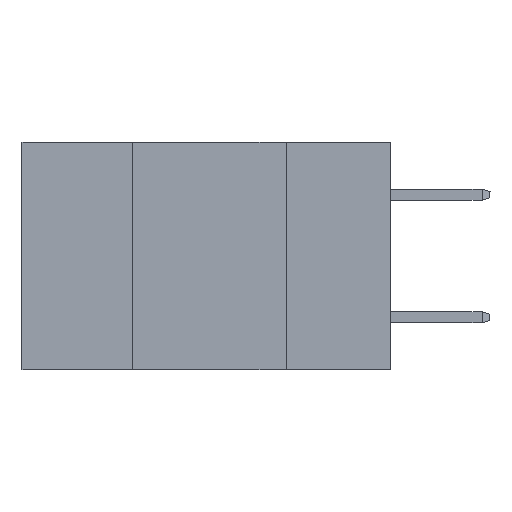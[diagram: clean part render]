
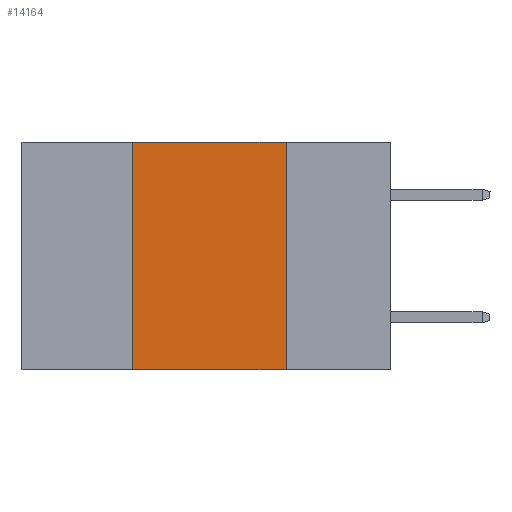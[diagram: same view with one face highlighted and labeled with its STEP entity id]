
A CAD part, left-side view. The second image highlights one B-rep face of the part: STEP entity #14164.
In plain terms, the highlighted planar face has unit normal (-1, 0, 0).
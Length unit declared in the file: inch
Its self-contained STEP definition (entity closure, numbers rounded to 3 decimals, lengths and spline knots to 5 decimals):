
#239 = DIRECTION ( 'NONE',  ( 0., 0., -1. ) ) ;
#480 = EDGE_LOOP ( 'NONE', ( #12639, #3311, #10027, #8172 ) ) ;
#546 = EDGE_CURVE ( 'NONE', #11624, #2412, #6965, .T. ) ;
#745 = CARTESIAN_POINT ( 'NONE',  ( 0., 0.42, -0.37 ) ) ;
#760 = DIRECTION ( 'NONE',  ( 0., -1., 0. ) ) ;
#1503 = DIRECTION ( 'NONE',  ( 0., -1., 0. ) ) ;
#1601 = EDGE_CURVE ( 'NONE', #4276, #13083, #14856, .T. ) ;
#2412 = VERTEX_POINT ( 'NONE', #15928 ) ;
#2461 = EDGE_CURVE ( 'NONE', #4276, #11624, #14995, .T. ) ;
#2687 = CARTESIAN_POINT ( 'NONE',  ( 0., 0.17, 0. ) ) ;
#3311 = ORIENTED_EDGE ( 'NONE', *, *, #546, .F. ) ;
#4276 = VERTEX_POINT ( 'NONE', #745 ) ;
#4395 = AXIS2_PLACEMENT_3D ( 'NONE', #5870, #10871, #4698 ) ;
#4698 = DIRECTION ( 'NONE',  ( 0., 0., -1. ) ) ;
#5870 = CARTESIAN_POINT ( 'NONE',  ( 0., 0.6, 0. ) ) ;
#6089 = CARTESIAN_POINT ( 'NONE',  ( 0., 0.42, 0. ) ) ;
#6965 = LINE ( 'NONE', #8244, #11828 ) ;
#8003 = VECTOR ( 'NONE', #760, 39.37008 ) ;
#8172 = ORIENTED_EDGE ( 'NONE', *, *, #1601, .T. ) ;
#8244 = CARTESIAN_POINT ( 'NONE',  ( 0., 0.6, 0. ) ) ;
#10027 = ORIENTED_EDGE ( 'NONE', *, *, #2461, .F. ) ;
#10190 = CARTESIAN_POINT ( 'NONE',  ( 0., 0.17, -0.37 ) ) ;
#10871 = DIRECTION ( 'NONE',  ( 1., 0., 0. ) ) ;
#11314 = VECTOR ( 'NONE', #12193, 39.37008 ) ;
#11624 = VERTEX_POINT ( 'NONE', #6089 ) ;
#11828 = VECTOR ( 'NONE', #1503, 39.37008 ) ;
#12193 = DIRECTION ( 'NONE',  ( 0., 0., 1. ) ) ;
#12218 = PLANE ( 'NONE',  #4395 ) ;
#12289 = CARTESIAN_POINT ( 'NONE',  ( 0., 0.42, 0. ) ) ;
#12460 = VECTOR ( 'NONE', #239, 39.37008 ) ;
#12639 = ORIENTED_EDGE ( 'NONE', *, *, #12776, .F. ) ;
#12776 = EDGE_CURVE ( 'NONE', #2412, #13083, #13240, .T. ) ;
#13083 = VERTEX_POINT ( 'NONE', #10190 ) ;
#13240 = LINE ( 'NONE', #2687, #12460 ) ;
#13415 = FACE_OUTER_BOUND ( 'NONE', #480, .T. ) ;
#14164 = ADVANCED_FACE ( 'NONE', ( #13415 ), #12218, .F. ) ;
#14856 = LINE ( 'NONE', #14950, #8003 ) ;
#14950 = CARTESIAN_POINT ( 'NONE',  ( 0., 0.6, -0.37 ) ) ;
#14995 = LINE ( 'NONE', #12289, #11314 ) ;
#15928 = CARTESIAN_POINT ( 'NONE',  ( 0., 0.17, 0. ) ) ;
